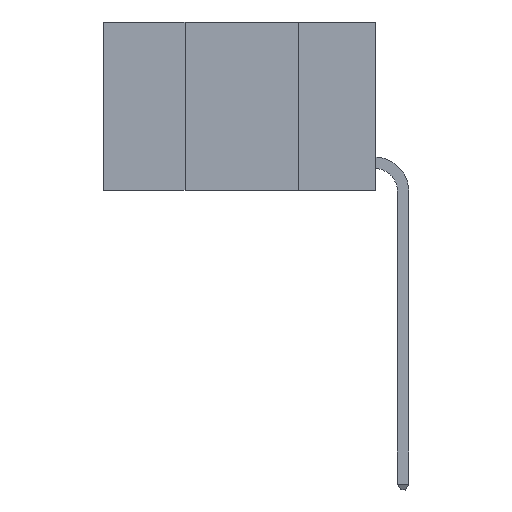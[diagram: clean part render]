
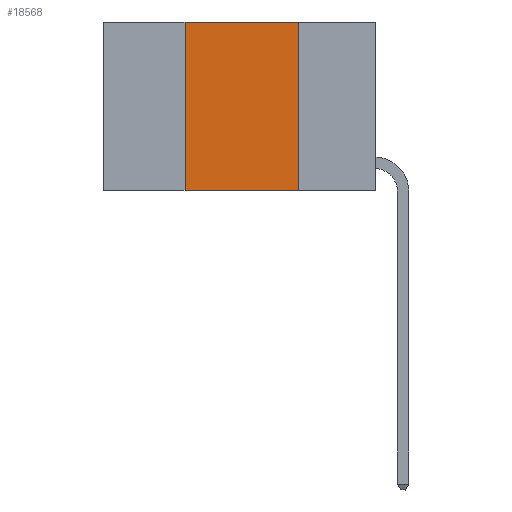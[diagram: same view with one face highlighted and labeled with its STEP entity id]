
A CAD part, left-side view. The second image highlights one B-rep face of the part: STEP entity #18568.
In plain terms, the highlighted planar face has unit normal (-1, 0, 0).
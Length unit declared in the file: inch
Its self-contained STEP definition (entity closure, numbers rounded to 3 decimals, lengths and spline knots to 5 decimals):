
#555 = EDGE_CURVE ( 'NONE', #17215, #11307, #15821, .T. ) ;
#1202 = CARTESIAN_POINT ( 'NONE',  ( 0., 0.6, 0. ) ) ;
#1398 = CARTESIAN_POINT ( 'NONE',  ( 0., 0.42, -0.37 ) ) ;
#2624 = CARTESIAN_POINT ( 'NONE',  ( 0., 0.42, 0. ) ) ;
#2714 = DIRECTION ( 'NONE',  ( 0., 0., -1. ) ) ;
#2794 = CARTESIAN_POINT ( 'NONE',  ( 0., 0.17, -0.37 ) ) ;
#4256 = VECTOR ( 'NONE', #9940, 39.37008 ) ;
#4534 = VECTOR ( 'NONE', #7142, 39.37008 ) ;
#5156 = CARTESIAN_POINT ( 'NONE',  ( 0., 0.17, 0. ) ) ;
#5234 = EDGE_LOOP ( 'NONE', ( #5675, #9585, #15764, #11842 ) ) ;
#5675 = ORIENTED_EDGE ( 'NONE', *, *, #555, .F. ) ;
#6570 = EDGE_CURVE ( 'NONE', #9643, #17215, #16222, .T. ) ;
#6751 = AXIS2_PLACEMENT_3D ( 'NONE', #1202, #11497, #2714 ) ;
#7142 = DIRECTION ( 'NONE',  ( 0., -1., 0. ) ) ;
#7837 = CARTESIAN_POINT ( 'NONE',  ( 0., 0.6, -0.37 ) ) ;
#8069 = LINE ( 'NONE', #7837, #11459 ) ;
#8291 = EDGE_CURVE ( 'NONE', #18630, #9643, #15511, .T. ) ;
#9272 = EDGE_CURVE ( 'NONE', #18630, #11307, #8069, .T. ) ;
#9552 = DIRECTION ( 'NONE',  ( 0., 0., -1. ) ) ;
#9585 = ORIENTED_EDGE ( 'NONE', *, *, #6570, .F. ) ;
#9643 = VERTEX_POINT ( 'NONE', #2624 ) ;
#9940 = DIRECTION ( 'NONE',  ( 0., 0., 1. ) ) ;
#11307 = VERTEX_POINT ( 'NONE', #2794 ) ;
#11459 = VECTOR ( 'NONE', #12200, 39.37008 ) ;
#11497 = DIRECTION ( 'NONE',  ( 1., 0., 0. ) ) ;
#11842 = ORIENTED_EDGE ( 'NONE', *, *, #9272, .T. ) ;
#11901 = VECTOR ( 'NONE', #9552, 39.37008 ) ;
#12200 = DIRECTION ( 'NONE',  ( 0., -1., 0. ) ) ;
#12840 = CARTESIAN_POINT ( 'NONE',  ( 0., 0.17, 0. ) ) ;
#14426 = CARTESIAN_POINT ( 'NONE',  ( 0., 0.6, 0. ) ) ;
#15452 = FACE_OUTER_BOUND ( 'NONE', #5234, .T. ) ;
#15511 = LINE ( 'NONE', #18644, #4256 ) ;
#15764 = ORIENTED_EDGE ( 'NONE', *, *, #8291, .F. ) ;
#15821 = LINE ( 'NONE', #5156, #11901 ) ;
#16222 = LINE ( 'NONE', #14426, #4534 ) ;
#17215 = VERTEX_POINT ( 'NONE', #12840 ) ;
#17296 = PLANE ( 'NONE',  #6751 ) ;
#18568 = ADVANCED_FACE ( 'NONE', ( #15452 ), #17296, .F. ) ;
#18630 = VERTEX_POINT ( 'NONE', #1398 ) ;
#18644 = CARTESIAN_POINT ( 'NONE',  ( 0., 0.42, 0. ) ) ;
